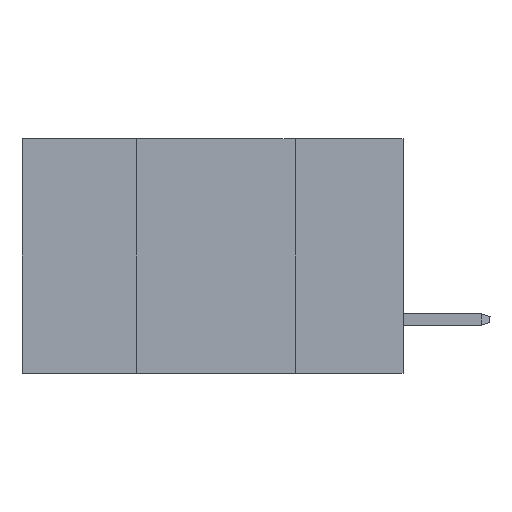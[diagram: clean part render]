
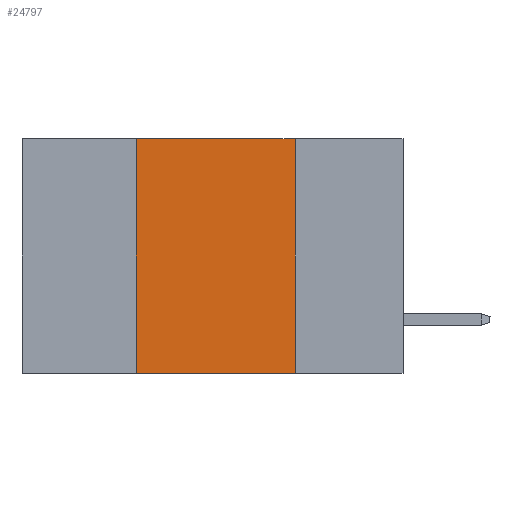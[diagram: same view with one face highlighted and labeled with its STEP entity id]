
A CAD part, left-side view. The second image highlights one B-rep face of the part: STEP entity #24797.
In plain terms, the highlighted planar face has unit normal (-1, 0, 0).
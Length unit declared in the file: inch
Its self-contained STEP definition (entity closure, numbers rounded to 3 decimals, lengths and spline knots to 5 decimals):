
#868 = LINE ( 'NONE', #1004, #3281 ) ;
#1004 = CARTESIAN_POINT ( 'NONE',  ( 0., 0.17, 0. ) ) ;
#2093 = CARTESIAN_POINT ( 'NONE',  ( 0., 0.42, 0. ) ) ;
#2511 = PLANE ( 'NONE',  #17915 ) ;
#2702 = VECTOR ( 'NONE', #12235, 39.37008 ) ;
#3281 = VECTOR ( 'NONE', #7380, 39.37008 ) ;
#3600 = LINE ( 'NONE', #24366, #22943 ) ;
#6129 = CARTESIAN_POINT ( 'NONE',  ( 0., 0.42, -0.37 ) ) ;
#6586 = DIRECTION ( 'NONE',  ( 1., 0., 0. ) ) ;
#7380 = DIRECTION ( 'NONE',  ( 0., 0., -1. ) ) ;
#8496 = ORIENTED_EDGE ( 'NONE', *, *, #9852, .F. ) ;
#8585 = ORIENTED_EDGE ( 'NONE', *, *, #14928, .T. ) ;
#9330 = VECTOR ( 'NONE', #10254, 39.37008 ) ;
#9852 = EDGE_CURVE ( 'NONE', #22590, #26245, #20714, .T. ) ;
#10254 = DIRECTION ( 'NONE',  ( 0., 0., 1. ) ) ;
#10789 = CARTESIAN_POINT ( 'NONE',  ( 0., 0.6, 0. ) ) ;
#11031 = CARTESIAN_POINT ( 'NONE',  ( 0., 0.17, -0.37 ) ) ;
#11509 = EDGE_CURVE ( 'NONE', #26245, #22519, #3600, .T. ) ;
#12235 = DIRECTION ( 'NONE',  ( 0., -1., 0. ) ) ;
#13344 = CARTESIAN_POINT ( 'NONE',  ( 0., 0.42, 0. ) ) ;
#13564 = EDGE_LOOP ( 'NONE', ( #25317, #14628, #8496, #8585 ) ) ;
#14628 = ORIENTED_EDGE ( 'NONE', *, *, #11509, .F. ) ;
#14928 = EDGE_CURVE ( 'NONE', #22590, #23569, #20402, .T. ) ;
#16085 = DIRECTION ( 'NONE',  ( 0., -1., 0. ) ) ;
#17915 = AXIS2_PLACEMENT_3D ( 'NONE', #10789, #6586, #18838 ) ;
#18838 = DIRECTION ( 'NONE',  ( 0., 0., -1. ) ) ;
#19996 = CARTESIAN_POINT ( 'NONE',  ( 0., 0.6, -0.37 ) ) ;
#20402 = LINE ( 'NONE', #19996, #2702 ) ;
#20714 = LINE ( 'NONE', #2093, #9330 ) ;
#21382 = FACE_OUTER_BOUND ( 'NONE', #13564, .T. ) ;
#21863 = EDGE_CURVE ( 'NONE', #22519, #23569, #868, .T. ) ;
#22519 = VERTEX_POINT ( 'NONE', #23093 ) ;
#22590 = VERTEX_POINT ( 'NONE', #6129 ) ;
#22943 = VECTOR ( 'NONE', #16085, 39.37008 ) ;
#23093 = CARTESIAN_POINT ( 'NONE',  ( 0., 0.17, 0. ) ) ;
#23569 = VERTEX_POINT ( 'NONE', #11031 ) ;
#24366 = CARTESIAN_POINT ( 'NONE',  ( 0., 0.6, 0. ) ) ;
#24797 = ADVANCED_FACE ( 'NONE', ( #21382 ), #2511, .F. ) ;
#25317 = ORIENTED_EDGE ( 'NONE', *, *, #21863, .F. ) ;
#26245 = VERTEX_POINT ( 'NONE', #13344 ) ;
